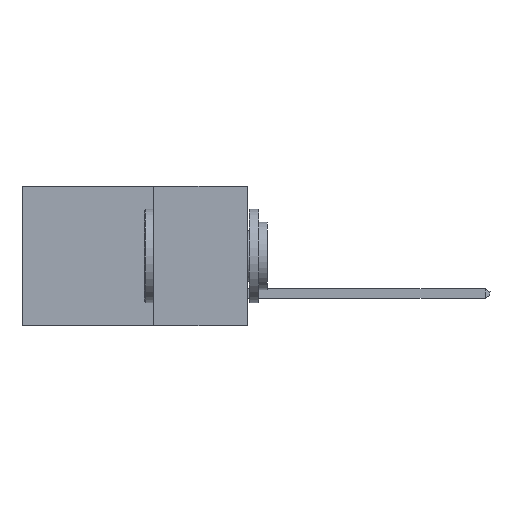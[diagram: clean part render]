
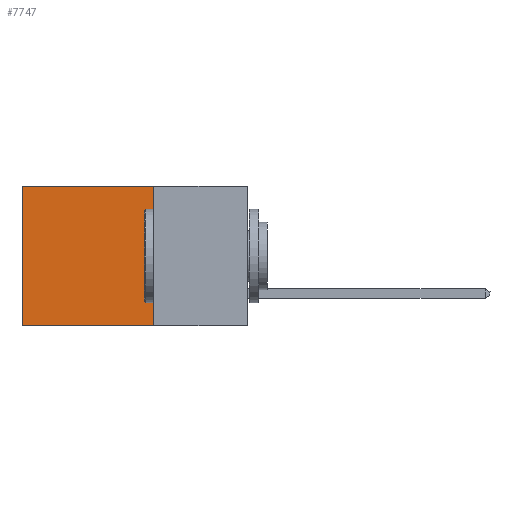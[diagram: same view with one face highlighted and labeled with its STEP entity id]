
A CAD part, left-side view. The second image highlights one B-rep face of the part: STEP entity #7747.
In plain terms, the highlighted planar face has unit normal (-1, 0, 0).
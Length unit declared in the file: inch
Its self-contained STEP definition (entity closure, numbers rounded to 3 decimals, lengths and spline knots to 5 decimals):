
#284 = VECTOR ( 'NONE', #5473, 39.37008 ) ;
#390 = DIRECTION ( 'NONE',  ( 0., 0., -1. ) ) ;
#621 = ORIENTED_EDGE ( 'NONE', *, *, #2011, .F. ) ;
#822 = DIRECTION ( 'NONE',  ( 1., 0., 0. ) ) ;
#1261 = DIRECTION ( 'NONE',  ( 0., 1., 0. ) ) ;
#1642 = VECTOR ( 'NONE', #390, 39.37008 ) ;
#1643 = PLANE ( 'NONE',  #10798 ) ;
#1693 = EDGE_CURVE ( 'NONE', #7938, #4315, #3647, .T. ) ;
#2011 = EDGE_CURVE ( 'NONE', #7938, #4398, #3712, .T. ) ;
#2153 = ORIENTED_EDGE ( 'NONE', *, *, #2527, .T. ) ;
#2172 = CARTESIAN_POINT ( 'NONE',  ( 0.2615, 0.6, 0. ) ) ;
#2365 = ORIENTED_EDGE ( 'NONE', *, *, #1693, .T. ) ;
#2527 = EDGE_CURVE ( 'NONE', #4315, #5498, #9936, .T. ) ;
#3647 = LINE ( 'NONE', #4489, #10428 ) ;
#3712 = LINE ( 'NONE', #8887, #1642 ) ;
#4253 = DIRECTION ( 'NONE',  ( 0., 0., -1. ) ) ;
#4315 = VERTEX_POINT ( 'NONE', #2172 ) ;
#4398 = VERTEX_POINT ( 'NONE', #7450 ) ;
#4489 = CARTESIAN_POINT ( 'NONE',  ( 0.2615, 0.25, 0. ) ) ;
#4649 = LINE ( 'NONE', #9592, #5572 ) ;
#5473 = DIRECTION ( 'NONE',  ( 0., 0., -1. ) ) ;
#5498 = VERTEX_POINT ( 'NONE', #10551 ) ;
#5572 = VECTOR ( 'NONE', #1261, 39.37008 ) ;
#6604 = ORIENTED_EDGE ( 'NONE', *, *, #7934, .F. ) ;
#6845 = EDGE_LOOP ( 'NONE', ( #2153, #6604, #621, #2365 ) ) ;
#7028 = DIRECTION ( 'NONE',  ( 0., 1., 0. ) ) ;
#7450 = CARTESIAN_POINT ( 'NONE',  ( 0.2615, 0.25, -0.37 ) ) ;
#7747 = ADVANCED_FACE ( 'NONE', ( #8315 ), #1643, .F. ) ;
#7934 = EDGE_CURVE ( 'NONE', #4398, #5498, #4649, .T. ) ;
#7938 = VERTEX_POINT ( 'NONE', #8931 ) ;
#8315 = FACE_OUTER_BOUND ( 'NONE', #6845, .T. ) ;
#8366 = CARTESIAN_POINT ( 'NONE',  ( 0.2615, 0.25, -0.37 ) ) ;
#8834 = CARTESIAN_POINT ( 'NONE',  ( 0.2615, 0.6, -0.37 ) ) ;
#8887 = CARTESIAN_POINT ( 'NONE',  ( 0.2615, 0.25, -0.37 ) ) ;
#8931 = CARTESIAN_POINT ( 'NONE',  ( 0.2615, 0.25, 0. ) ) ;
#9592 = CARTESIAN_POINT ( 'NONE',  ( 0.2615, 0.25, -0.37 ) ) ;
#9936 = LINE ( 'NONE', #8834, #284 ) ;
#10428 = VECTOR ( 'NONE', #7028, 39.37008 ) ;
#10551 = CARTESIAN_POINT ( 'NONE',  ( 0.2615, 0.6, -0.37 ) ) ;
#10798 = AXIS2_PLACEMENT_3D ( 'NONE', #8366, #822, #4253 ) ;
